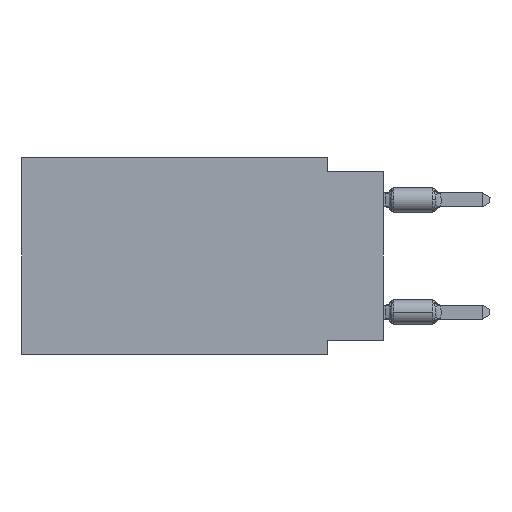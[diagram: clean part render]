
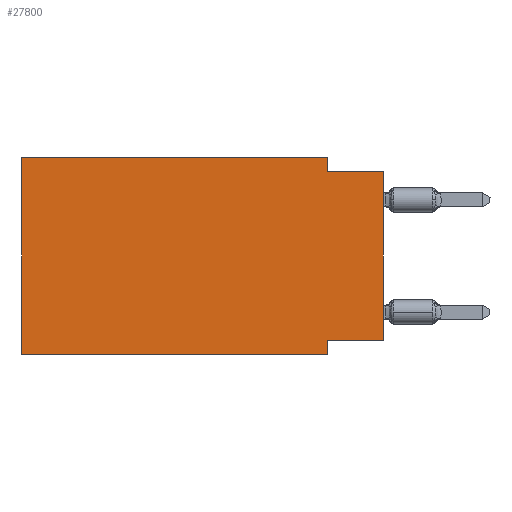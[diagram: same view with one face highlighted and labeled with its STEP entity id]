
A CAD part, left-side view. The second image highlights one B-rep face of the part: STEP entity #27800.
In plain terms, the highlighted planar face has unit normal (-1, 0, 0).
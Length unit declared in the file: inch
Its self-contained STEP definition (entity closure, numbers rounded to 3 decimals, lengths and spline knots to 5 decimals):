
#146 = VERTEX_POINT ( 'NONE', #33984 ) ;
#182 = DIRECTION ( 'NONE',  ( 0., -1., 0. ) ) ;
#349 = VECTOR ( 'NONE', #4322, 39.37008 ) ;
#2021 = VECTOR ( 'NONE', #182, 39.37008 ) ;
#3745 = ORIENTED_EDGE ( 'NONE', *, *, #11679, .T. ) ;
#4035 = EDGE_CURVE ( 'NONE', #146, #16294, #10183, .T. ) ;
#4322 = DIRECTION ( 'NONE',  ( 0., -1., 0. ) ) ;
#5066 = CARTESIAN_POINT ( 'NONE',  ( 0., 0.645, 0. ) ) ;
#6767 = DIRECTION ( 'NONE',  ( 0., 0., 1. ) ) ;
#7066 = EDGE_CURVE ( 'NONE', #7674, #30440, #25022, .T. ) ;
#7674 = VERTEX_POINT ( 'NONE', #30426 ) ;
#7831 = VECTOR ( 'NONE', #24813, 39.37008 ) ;
#8191 = FACE_OUTER_BOUND ( 'NONE', #20253, .T. ) ;
#9765 = VERTEX_POINT ( 'NONE', #22462 ) ;
#10183 = LINE ( 'NONE', #23639, #2021 ) ;
#11302 = DIRECTION ( 'NONE',  ( 1., 0., 0. ) ) ;
#11679 = EDGE_CURVE ( 'NONE', #41945, #16294, #23099, .T. ) ;
#11743 = DIRECTION ( 'NONE',  ( 0., 0., -1. ) ) ;
#13304 = AXIS2_PLACEMENT_3D ( 'NONE', #5066, #11302, #11743 ) ;
#14379 = CARTESIAN_POINT ( 'NONE',  ( 0., 0., -0.325 ) ) ;
#14864 = ORIENTED_EDGE ( 'NONE', *, *, #4035, .F. ) ;
#15727 = ORIENTED_EDGE ( 'NONE', *, *, #42533, .F. ) ;
#16042 = DIRECTION ( 'NONE',  ( 0., 0., 1. ) ) ;
#16043 = LINE ( 'NONE', #19575, #28057 ) ;
#16294 = VERTEX_POINT ( 'NONE', #40364 ) ;
#16368 = CARTESIAN_POINT ( 'NONE',  ( 0., 0.1, 0. ) ) ;
#17697 = DIRECTION ( 'NONE',  ( 0., 1., 0. ) ) ;
#18541 = VECTOR ( 'NONE', #16042, 39.37008 ) ;
#19575 = CARTESIAN_POINT ( 'NONE',  ( 0., 0.1, 0. ) ) ;
#20253 = EDGE_LOOP ( 'NONE', ( #3745, #14864, #15727, #41864, #31201, #32696, #28479, #34996 ) ) ;
#20523 = EDGE_CURVE ( 'NONE', #9765, #30440, #34563, .T. ) ;
#20570 = EDGE_CURVE ( 'NONE', #34837, #22517, #41642, .T. ) ;
#21776 = CARTESIAN_POINT ( 'NONE',  ( 0., 0.645, 0. ) ) ;
#22230 = VECTOR ( 'NONE', #31705, 39.37008 ) ;
#22462 = CARTESIAN_POINT ( 'NONE',  ( 0., 0.645, -0.35 ) ) ;
#22517 = VERTEX_POINT ( 'NONE', #16368 ) ;
#23099 = LINE ( 'NONE', #30343, #18541 ) ;
#23102 = DIRECTION ( 'NONE',  ( 0., 0., -1. ) ) ;
#23559 = CARTESIAN_POINT ( 'NONE',  ( 0., 0.1, -0.35 ) ) ;
#23639 = CARTESIAN_POINT ( 'NONE',  ( 0., 0., -0.025 ) ) ;
#23963 = CARTESIAN_POINT ( 'NONE',  ( 0., 0., -0.325 ) ) ;
#24813 = DIRECTION ( 'NONE',  ( 0., 0., -1. ) ) ;
#25022 = LINE ( 'NONE', #38026, #7831 ) ;
#27800 = ADVANCED_FACE ( 'NONE', ( #8191 ), #41520, .F. ) ;
#28057 = VECTOR ( 'NONE', #23102, 39.37008 ) ;
#28479 = ORIENTED_EDGE ( 'NONE', *, *, #7066, .F. ) ;
#30343 = CARTESIAN_POINT ( 'NONE',  ( 0., 0., 0. ) ) ;
#30426 = CARTESIAN_POINT ( 'NONE',  ( 0., 0.1, -0.325 ) ) ;
#30440 = VERTEX_POINT ( 'NONE', #23559 ) ;
#31201 = ORIENTED_EDGE ( 'NONE', *, *, #41362, .F. ) ;
#31347 = LINE ( 'NONE', #14379, #38772 ) ;
#31474 = CARTESIAN_POINT ( 'NONE',  ( 0., 0.645, -0.35 ) ) ;
#31705 = DIRECTION ( 'NONE',  ( 0., -1., 0. ) ) ;
#32696 = ORIENTED_EDGE ( 'NONE', *, *, #20523, .T. ) ;
#33300 = EDGE_CURVE ( 'NONE', #41945, #7674, #31347, .T. ) ;
#33984 = CARTESIAN_POINT ( 'NONE',  ( 0., 0.1, -0.025 ) ) ;
#34563 = LINE ( 'NONE', #31474, #349 ) ;
#34837 = VERTEX_POINT ( 'NONE', #42865 ) ;
#34996 = ORIENTED_EDGE ( 'NONE', *, *, #33300, .F. ) ;
#35846 = VECTOR ( 'NONE', #6767, 39.37008 ) ;
#37238 = LINE ( 'NONE', #43625, #35846 ) ;
#38026 = CARTESIAN_POINT ( 'NONE',  ( 0., 0.1, -0.35 ) ) ;
#38772 = VECTOR ( 'NONE', #17697, 39.37008 ) ;
#40364 = CARTESIAN_POINT ( 'NONE',  ( 0., 0., -0.025 ) ) ;
#41362 = EDGE_CURVE ( 'NONE', #9765, #34837, #37238, .T. ) ;
#41520 = PLANE ( 'NONE',  #13304 ) ;
#41642 = LINE ( 'NONE', #21776, #22230 ) ;
#41864 = ORIENTED_EDGE ( 'NONE', *, *, #20570, .F. ) ;
#41945 = VERTEX_POINT ( 'NONE', #23963 ) ;
#42533 = EDGE_CURVE ( 'NONE', #22517, #146, #16043, .T. ) ;
#42865 = CARTESIAN_POINT ( 'NONE',  ( 0., 0.645, 0. ) ) ;
#43625 = CARTESIAN_POINT ( 'NONE',  ( 0., 0.645, 0. ) ) ;
